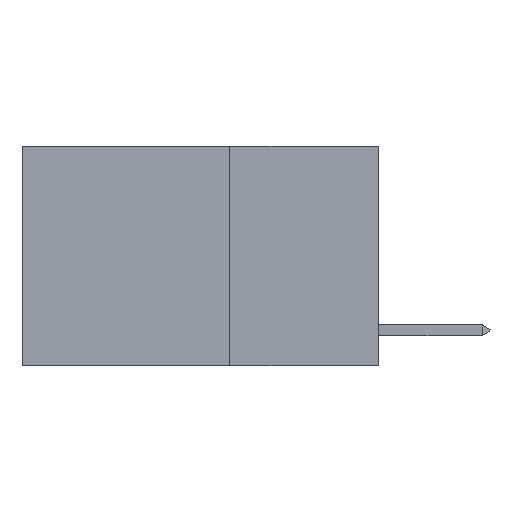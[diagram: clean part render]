
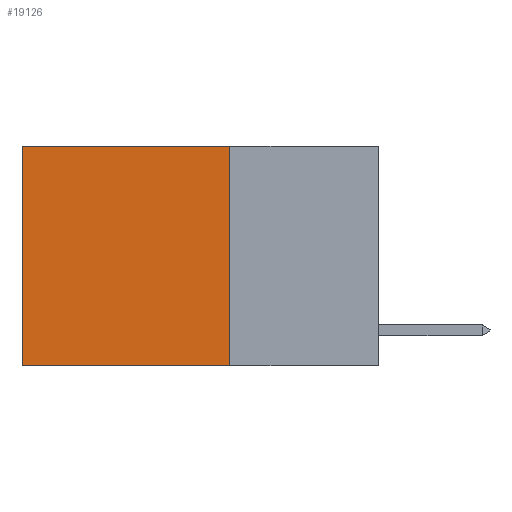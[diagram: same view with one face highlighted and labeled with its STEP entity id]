
A CAD part, left-side view. The second image highlights one B-rep face of the part: STEP entity #19126.
In plain terms, the highlighted planar face has unit normal (-1, 0, 0).
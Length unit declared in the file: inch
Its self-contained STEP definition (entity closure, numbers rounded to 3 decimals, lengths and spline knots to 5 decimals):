
#952 = CARTESIAN_POINT ( 'NONE',  ( 0.2625, 0.25, 0. ) ) ;
#1465 = CARTESIAN_POINT ( 'NONE',  ( 0.2625, 0.25, 0. ) ) ;
#1609 = LINE ( 'NONE', #11030, #22138 ) ;
#3223 = VERTEX_POINT ( 'NONE', #17634 ) ;
#3379 = VECTOR ( 'NONE', #8426, 39.37008 ) ;
#5325 = VECTOR ( 'NONE', #23730, 39.37008 ) ;
#8229 = DIRECTION ( 'NONE',  ( 0., 0., -1. ) ) ;
#8426 = DIRECTION ( 'NONE',  ( 0., 1., 0. ) ) ;
#9948 = AXIS2_PLACEMENT_3D ( 'NONE', #29406, #13044, #22955 ) ;
#11030 = CARTESIAN_POINT ( 'NONE',  ( 0.2625, 0.6, 0. ) ) ;
#13044 = DIRECTION ( 'NONE',  ( 1., 0., 0. ) ) ;
#13533 = EDGE_CURVE ( 'NONE', #21634, #20381, #17222, .T. ) ;
#14275 = VECTOR ( 'NONE', #8229, 39.37008 ) ;
#14947 = CARTESIAN_POINT ( 'NONE',  ( 0.2625, 0.6, -0.37 ) ) ;
#15105 = EDGE_CURVE ( 'NONE', #3223, #15259, #22647, .T. ) ;
#15259 = VERTEX_POINT ( 'NONE', #21698 ) ;
#16922 = CARTESIAN_POINT ( 'NONE',  ( 0.2625, 0.25, -0.37 ) ) ;
#17222 = LINE ( 'NONE', #16922, #5325 ) ;
#17634 = CARTESIAN_POINT ( 'NONE',  ( 0.2625, 0.25, 0. ) ) ;
#17852 = FACE_OUTER_BOUND ( 'NONE', #20586, .T. ) ;
#18857 = ORIENTED_EDGE ( 'NONE', *, *, #28310, .F. ) ;
#19126 = ADVANCED_FACE ( 'NONE', ( #17852 ), #22505, .F. ) ;
#19827 = LINE ( 'NONE', #952, #14275 ) ;
#20381 = VERTEX_POINT ( 'NONE', #14947 ) ;
#20459 = DIRECTION ( 'NONE',  ( 0., 0., -1. ) ) ;
#20586 = EDGE_LOOP ( 'NONE', ( #26148, #22676, #18857, #23573 ) ) ;
#21634 = VERTEX_POINT ( 'NONE', #26927 ) ;
#21698 = CARTESIAN_POINT ( 'NONE',  ( 0.2625, 0.6, 0. ) ) ;
#22138 = VECTOR ( 'NONE', #20459, 39.37008 ) ;
#22505 = PLANE ( 'NONE',  #9948 ) ;
#22647 = LINE ( 'NONE', #1465, #3379 ) ;
#22676 = ORIENTED_EDGE ( 'NONE', *, *, #13533, .F. ) ;
#22955 = DIRECTION ( 'NONE',  ( 0., 0., -1. ) ) ;
#23573 = ORIENTED_EDGE ( 'NONE', *, *, #15105, .T. ) ;
#23730 = DIRECTION ( 'NONE',  ( 0., 1., 0. ) ) ;
#26148 = ORIENTED_EDGE ( 'NONE', *, *, #26748, .T. ) ;
#26748 = EDGE_CURVE ( 'NONE', #15259, #20381, #1609, .T. ) ;
#26927 = CARTESIAN_POINT ( 'NONE',  ( 0.2625, 0.25, -0.37 ) ) ;
#28310 = EDGE_CURVE ( 'NONE', #3223, #21634, #19827, .T. ) ;
#29406 = CARTESIAN_POINT ( 'NONE',  ( 0.2625, 0.25, 0. ) ) ;
